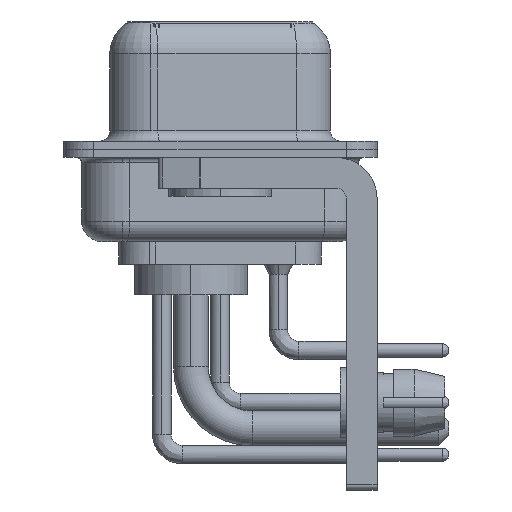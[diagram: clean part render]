
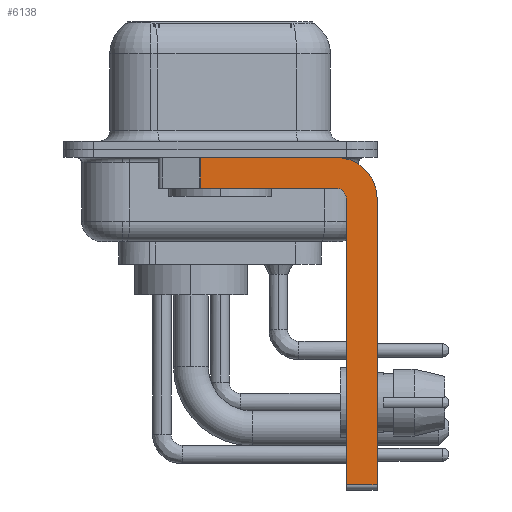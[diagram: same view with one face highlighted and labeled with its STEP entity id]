
A CAD part, left-side view. The second image highlights one B-rep face of the part: STEP entity #6138.
In plain terms, the highlighted planar face has unit normal (-1, 0, 0).
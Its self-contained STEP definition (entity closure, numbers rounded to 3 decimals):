
#1039 = DIRECTION ( 'NONE',  ( 0., 0., 1. ) ) ;
#2219 = EDGE_CURVE ( 'NONE', #20745, #4281, #31309, .T. ) ;
#2545 = EDGE_CURVE ( 'NONE', #22396, #7778, #7908, .T. ) ;
#3344 = ORIENTED_EDGE ( 'NONE', *, *, #31159, .F. ) ;
#3639 = AXIS2_PLACEMENT_3D ( 'NONE', #24537, #25229, #1039 ) ;
#4281 = VERTEX_POINT ( 'NONE', #9088 ) ;
#4333 = CARTESIAN_POINT ( 'NONE',  ( -2.9, -7.65, -2.4 ) ) ;
#4512 = CARTESIAN_POINT ( 'NONE',  ( -2.9, -5.65, -1.9 ) ) ;
#4857 = ORIENTED_EDGE ( 'NONE', *, *, #29722, .F. ) ;
#5330 = DIRECTION ( 'NONE',  ( 0., 0., -1. ) ) ;
#5561 = LINE ( 'NONE', #30117, #21930 ) ;
#6138 = ADVANCED_FACE ( 'NONE', ( #6438 ), #31295, .F. ) ;
#6438 = FACE_OUTER_BOUND ( 'NONE', #18388, .T. ) ;
#6480 = CARTESIAN_POINT ( 'NONE',  ( -2.9, -6.15, -16.6 ) ) ;
#6709 = CARTESIAN_POINT ( 'NONE',  ( -2.9, -7.65, -2.4 ) ) ;
#7090 = DIRECTION ( 'NONE',  ( 0., 0., -1. ) ) ;
#7577 = VERTEX_POINT ( 'NONE', #18642 ) ;
#7778 = VERTEX_POINT ( 'NONE', #33082 ) ;
#7908 = LINE ( 'NONE', #10382, #27364 ) ;
#9088 = CARTESIAN_POINT ( 'NONE',  ( -2.9, -5.65, -1.9 ) ) ;
#9479 = ORIENTED_EDGE ( 'NONE', *, *, #27193, .T. ) ;
#10382 = CARTESIAN_POINT ( 'NONE',  ( -2.9, 3., -0.4 ) ) ;
#11183 = DIRECTION ( 'NONE',  ( 1., 0., 0. ) ) ;
#11235 = DIRECTION ( 'NONE',  ( 1., 0., 0. ) ) ;
#13367 = EDGE_CURVE ( 'NONE', #31763, #13577, #22432, .T. ) ;
#13449 = VECTOR ( 'NONE', #32554, 1000. ) ;
#13577 = VERTEX_POINT ( 'NONE', #28945 ) ;
#13708 = VECTOR ( 'NONE', #21670, 1000. ) ;
#14382 = VERTEX_POINT ( 'NONE', #33134 ) ;
#15958 = ORIENTED_EDGE ( 'NONE', *, *, #2545, .F. ) ;
#16718 = CARTESIAN_POINT ( 'NONE',  ( -2.9, 0.978, -0.4 ) ) ;
#16930 = LINE ( 'NONE', #6480, #20367 ) ;
#17229 = CARTESIAN_POINT ( 'NONE',  ( -2.9, -5.65, -2.4 ) ) ;
#18388 = EDGE_LOOP ( 'NONE', ( #15958, #9479, #3344, #30508, #4857, #29938, #25458, #28295 ) ) ;
#18642 = CARTESIAN_POINT ( 'NONE',  ( -2.9, 0.978, -1.9 ) ) ;
#19408 = AXIS2_PLACEMENT_3D ( 'NONE', #17229, #11235, #7090 ) ;
#19479 = LINE ( 'NONE', #24063, #13449 ) ;
#19627 = DIRECTION ( 'NONE',  ( 0., 0., -1. ) ) ;
#20203 = AXIS2_PLACEMENT_3D ( 'NONE', #27230, #11183, #5330 ) ;
#20367 = VECTOR ( 'NONE', #27669, 1000. ) ;
#20616 = LINE ( 'NONE', #4512, #13708 ) ;
#20745 = VERTEX_POINT ( 'NONE', #25886 ) ;
#21517 = DIRECTION ( 'NONE',  ( 0., -1., 0. ) ) ;
#21670 = DIRECTION ( 'NONE',  ( 0., 1., 0. ) ) ;
#21930 = VECTOR ( 'NONE', #29781, 1000. ) ;
#22396 = VERTEX_POINT ( 'NONE', #16718 ) ;
#22432 = LINE ( 'NONE', #6709, #30852 ) ;
#24063 = CARTESIAN_POINT ( 'NONE',  ( -2.9, 0.978, -1.9 ) ) ;
#24537 = CARTESIAN_POINT ( 'NONE',  ( -2.9, -5.65, -2.4 ) ) ;
#25229 = DIRECTION ( 'NONE',  ( -1., 0., 0. ) ) ;
#25458 = ORIENTED_EDGE ( 'NONE', *, *, #13367, .F. ) ;
#25886 = CARTESIAN_POINT ( 'NONE',  ( -2.9, -6.15, -2.4 ) ) ;
#27193 = EDGE_CURVE ( 'NONE', #22396, #7577, #19479, .T. ) ;
#27230 = CARTESIAN_POINT ( 'NONE',  ( -2.9, -5.65, -2.4 ) ) ;
#27238 = EDGE_CURVE ( 'NONE', #7778, #31763, #30338, .T. ) ;
#27364 = VECTOR ( 'NONE', #21517, 1000. ) ;
#27669 = DIRECTION ( 'NONE',  ( 0., 0., 1. ) ) ;
#28080 = EDGE_CURVE ( 'NONE', #14382, #13577, #5561, .T. ) ;
#28295 = ORIENTED_EDGE ( 'NONE', *, *, #27238, .F. ) ;
#28945 = CARTESIAN_POINT ( 'NONE',  ( -2.9, -7.65, -16.35 ) ) ;
#29722 = EDGE_CURVE ( 'NONE', #14382, #20745, #16930, .T. ) ;
#29781 = DIRECTION ( 'NONE',  ( 0., -1., 0. ) ) ;
#29938 = ORIENTED_EDGE ( 'NONE', *, *, #28080, .T. ) ;
#30117 = CARTESIAN_POINT ( 'NONE',  ( -2.9, -5.65, -16.35 ) ) ;
#30338 = CIRCLE ( 'NONE', #20203, 2. ) ;
#30508 = ORIENTED_EDGE ( 'NONE', *, *, #2219, .F. ) ;
#30852 = VECTOR ( 'NONE', #19627, 1000. ) ;
#31159 = EDGE_CURVE ( 'NONE', #4281, #7577, #20616, .T. ) ;
#31295 = PLANE ( 'NONE',  #19408 ) ;
#31309 = CIRCLE ( 'NONE', #3639, 0.5 ) ;
#31763 = VERTEX_POINT ( 'NONE', #4333 ) ;
#32554 = DIRECTION ( 'NONE',  ( 0., 0., -1. ) ) ;
#33082 = CARTESIAN_POINT ( 'NONE',  ( -2.9, -5.65, -0.4 ) ) ;
#33134 = CARTESIAN_POINT ( 'NONE',  ( -2.9, -6.15, -16.35 ) ) ;
